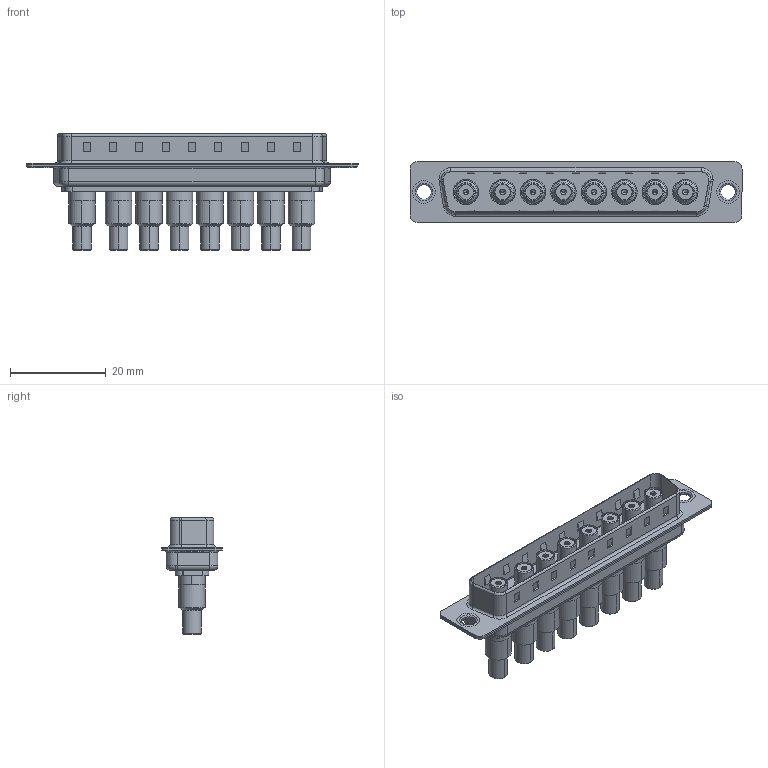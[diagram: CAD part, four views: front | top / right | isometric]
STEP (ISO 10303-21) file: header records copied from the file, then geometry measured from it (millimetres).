
FILE_DESCRIPTION (( 'STEP AP203' ), '1' );
FILE_NAME ('627-8W8-222-5N1.STEP', '2019-05-28T03:01:57', ( '' ), ( '' ), 'SwSTEP 2.0', 'SolidWorks 2016', '' );
FILE_SCHEMA (( 'CONFIG_CONTROL_DESIGN' ));
Length unit declared in the file: millimetre
Products named in the file (12): 627Combo Shell Front_37 Contacts; Insulator Socket; 627Combo Thru Hole Rivet; 627-8W8-222-5N1; Co-Ax Jack_Solder Cup Tail; Socket_Solder Cup; Solder Cover; Locking Collar; Insulator Socket 2; 627Combo Housing_8W8; 627Combo Shell Rear_37 Contacts; Co-Ax Jack Assy_SC
Assembly tree (19 placements, depth 3):
  627-8W8-222-5N1
    627Combo Housing_8W8
    627Combo Shell Rear_37 Contacts
    627Combo Shell Front_37 Contacts
    627Combo Thru Hole Rivet  x2
    Co-Ax Jack Assy_SC  x8
      Co-Ax Jack_Solder Cup Tail
      Insulator Socket
      Insulator Socket 2
      Locking Collar
      Socket_Solder Cup
      Solder Cover
Bounding box: 69.3 x 12.6 x 24.3 mm (x, y, z)
Volume: 4720 mm3; surface area: 15772.5 mm2
Topology: 53 solids, 53 shells, 1426 faces, 3287 edges, 2018 vertices
Faces by surface type: cylinder 637, plane 523, cone 160, torus 90, bspline 16
Entity records: 17425 total; most frequent: DIRECTION 2884, CARTESIAN_POINT 2864, ORIENTED_EDGE 2604, EDGE_CURVE 1302, AXIS2_PLACEMENT_3D 1059, VERTEX_POINT 818, LINE 766, VECTOR 766
